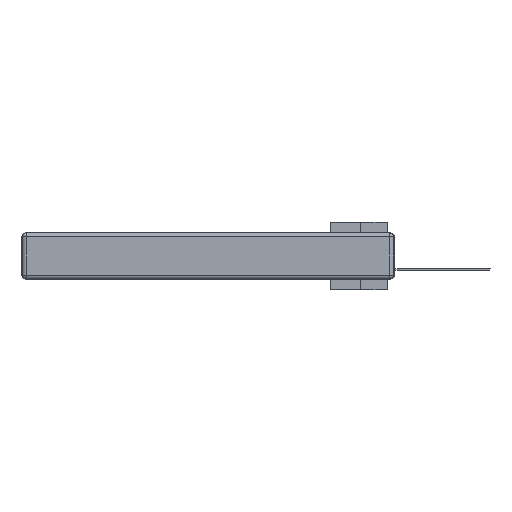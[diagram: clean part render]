
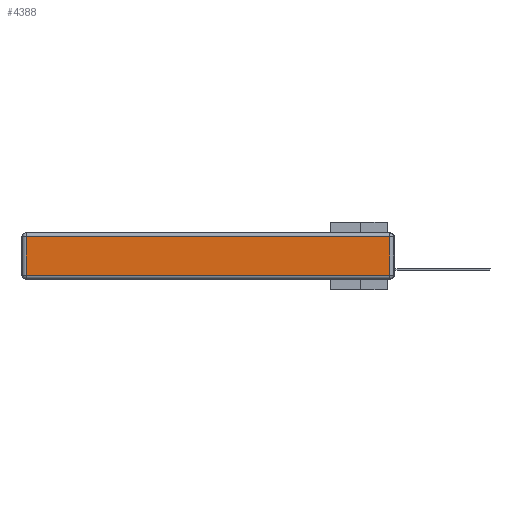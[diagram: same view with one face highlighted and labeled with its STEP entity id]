
A CAD part, left-side view. The second image highlights one B-rep face of the part: STEP entity #4388.
In plain terms, the highlighted planar face has unit normal (-1, 0, 0).
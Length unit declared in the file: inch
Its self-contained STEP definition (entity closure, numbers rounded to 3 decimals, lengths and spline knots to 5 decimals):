
#101 = VECTOR ( 'NONE', #10578, 39.37008 ) ;
#217 = ORIENTED_EDGE ( 'NONE', *, *, #923, .T. ) ;
#923 = EDGE_CURVE ( 'NONE', #25329, #9702, #1703, .T. ) ;
#1166 = VERTEX_POINT ( 'NONE', #23662 ) ;
#1703 = LINE ( 'NONE', #23165, #3141 ) ;
#2208 = VECTOR ( 'NONE', #29320, 39.37008 ) ;
#2299 = DIRECTION ( 'NONE',  ( -1., 0., 0. ) ) ;
#2403 = DIRECTION ( 'NONE',  ( 0., 0., 1. ) ) ;
#3139 = EDGE_CURVE ( 'NONE', #9702, #14435, #13477, .T. ) ;
#3141 = VECTOR ( 'NONE', #22860, 39.37008 ) ;
#3620 = ORIENTED_EDGE ( 'NONE', *, *, #28297, .T. ) ;
#4388 = ADVANCED_FACE ( 'NONE', ( #18475 ), #9260, .T. ) ;
#6454 = VECTOR ( 'NONE', #13493, 39.37008 ) ;
#6977 = CARTESIAN_POINT ( 'NONE',  ( 0., 0.03, -0.313 ) ) ;
#7325 = ORIENTED_EDGE ( 'NONE', *, *, #3139, .T. ) ;
#8446 = CARTESIAN_POINT ( 'NONE',  ( 0., 2.75, -0.03 ) ) ;
#9260 = PLANE ( 'NONE',  #12442 ) ;
#9702 = VERTEX_POINT ( 'NONE', #17581 ) ;
#9888 = ORIENTED_EDGE ( 'NONE', *, *, #17555, .T. ) ;
#10578 = DIRECTION ( 'NONE',  ( 0., 1., 0. ) ) ;
#12442 = AXIS2_PLACEMENT_3D ( 'NONE', #27730, #2299, #2403 ) ;
#13477 = LINE ( 'NONE', #8446, #101 ) ;
#13493 = DIRECTION ( 'NONE',  ( 0., 0., -1. ) ) ;
#13575 = CARTESIAN_POINT ( 'NONE',  ( 0., 0., -0.313 ) ) ;
#14435 = VERTEX_POINT ( 'NONE', #23847 ) ;
#17510 = CARTESIAN_POINT ( 'NONE',  ( 0., 2.72, -0.343 ) ) ;
#17555 = EDGE_CURVE ( 'NONE', #14435, #1166, #17996, .T. ) ;
#17581 = CARTESIAN_POINT ( 'NONE',  ( 0., 0.03, -0.03 ) ) ;
#17996 = LINE ( 'NONE', #17510, #6454 ) ;
#18475 = FACE_OUTER_BOUND ( 'NONE', #28734, .T. ) ;
#20252 = LINE ( 'NONE', #13575, #2208 ) ;
#22860 = DIRECTION ( 'NONE',  ( 0., 0., 1. ) ) ;
#23165 = CARTESIAN_POINT ( 'NONE',  ( 0., 0.03, -0.343 ) ) ;
#23662 = CARTESIAN_POINT ( 'NONE',  ( 0., 2.72, -0.313 ) ) ;
#23847 = CARTESIAN_POINT ( 'NONE',  ( 0., 2.72, -0.03 ) ) ;
#25329 = VERTEX_POINT ( 'NONE', #6977 ) ;
#27730 = CARTESIAN_POINT ( 'NONE',  ( 0., 0., -0.343 ) ) ;
#28297 = EDGE_CURVE ( 'NONE', #1166, #25329, #20252, .T. ) ;
#28734 = EDGE_LOOP ( 'NONE', ( #3620, #217, #7325, #9888 ) ) ;
#29320 = DIRECTION ( 'NONE',  ( 0., -1., 0. ) ) ;
